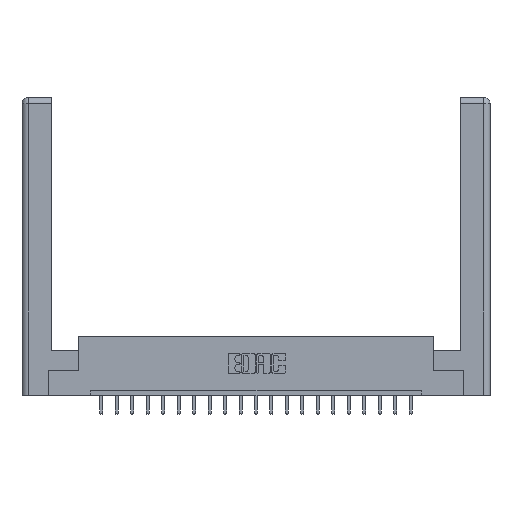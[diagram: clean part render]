
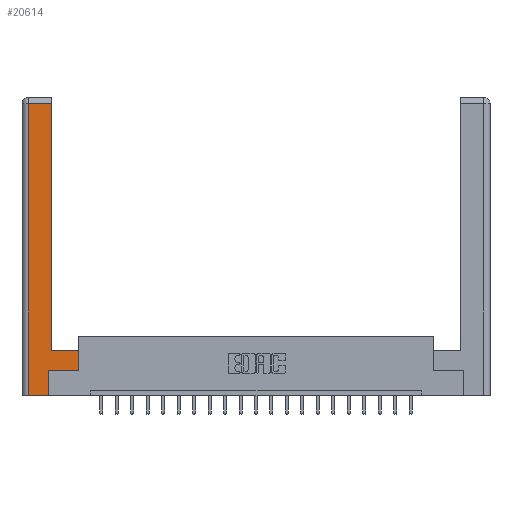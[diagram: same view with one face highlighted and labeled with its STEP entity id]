
A CAD part, top view. The second image highlights one B-rep face of the part: STEP entity #20614.
In plain terms, the highlighted planar face has unit normal (0, 0, 1).
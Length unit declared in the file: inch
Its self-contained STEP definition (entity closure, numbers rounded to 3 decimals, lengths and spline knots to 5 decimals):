
#14 = VERTEX_POINT ( 'NONE', #2744 ) ;
#139 = DIRECTION ( 'NONE',  ( 0., -1., 0. ) ) ;
#161 = LINE ( 'NONE', #10809, #4755 ) ;
#211 = CARTESIAN_POINT ( 'NONE',  ( 0.565, 0.245, 0. ) ) ;
#277 = ORIENTED_EDGE ( 'NONE', *, *, #19937, .T. ) ;
#769 = VERTEX_POINT ( 'NONE', #12745 ) ;
#966 = DIRECTION ( 'NONE',  ( 0., 1., 0. ) ) ;
#1201 = VECTOR ( 'NONE', #10895, 39.37008 ) ;
#1247 = EDGE_CURVE ( 'NONE', #20929, #9600, #13380, .T. ) ;
#1670 = EDGE_LOOP ( 'NONE', ( #7383, #277, #18911, #3865, #18417, #17178, #19690, #11444 ) ) ;
#2225 = VERTEX_POINT ( 'NONE', #3813 ) ;
#2557 = CARTESIAN_POINT ( 'NONE',  ( 0., 0., 0. ) ) ;
#2691 = VECTOR ( 'NONE', #9878, 39.37008 ) ;
#2744 = CARTESIAN_POINT ( 'NONE',  ( 0.0615, 0., 0. ) ) ;
#3380 = CARTESIAN_POINT ( 'NONE',  ( 0.265, 0.245, 0. ) ) ;
#3390 = AXIS2_PLACEMENT_3D ( 'NONE', #2557, #13781, #13850 ) ;
#3813 = CARTESIAN_POINT ( 'NONE',  ( 0.295, 0.45, 0. ) ) ;
#3865 = ORIENTED_EDGE ( 'NONE', *, *, #11251, .T. ) ;
#4700 = VECTOR ( 'NONE', #5051, 39.37008 ) ;
#4755 = VECTOR ( 'NONE', #5991, 39.37008 ) ;
#5001 = CARTESIAN_POINT ( 'NONE',  ( 0.0615, 2.94, 0. ) ) ;
#5007 = LINE ( 'NONE', #20557, #1201 ) ;
#5051 = DIRECTION ( 'NONE',  ( 1., 0., 0. ) ) ;
#5991 = DIRECTION ( 'NONE',  ( 1., 0., 0. ) ) ;
#7077 = DIRECTION ( 'NONE',  ( -1., 0., 0. ) ) ;
#7383 = ORIENTED_EDGE ( 'NONE', *, *, #8585, .T. ) ;
#8111 = EDGE_CURVE ( 'NONE', #16551, #2225, #19938, .T. ) ;
#8377 = CARTESIAN_POINT ( 'NONE',  ( 0.0615, 0., 0. ) ) ;
#8585 = EDGE_CURVE ( 'NONE', #2225, #769, #18625, .T. ) ;
#9307 = LINE ( 'NONE', #8377, #16709 ) ;
#9600 = VERTEX_POINT ( 'NONE', #16632 ) ;
#9878 = DIRECTION ( 'NONE',  ( 0., 1., 0. ) ) ;
#10134 = CARTESIAN_POINT ( 'NONE',  ( 0.265, 0., 0. ) ) ;
#10657 = CARTESIAN_POINT ( 'NONE',  ( 0.565, 0.45, 0. ) ) ;
#10809 = CARTESIAN_POINT ( 'NONE',  ( 0.265, 0., 0. ) ) ;
#10895 = DIRECTION ( 'NONE',  ( -1., 0., 0. ) ) ;
#11251 = EDGE_CURVE ( 'NONE', #14, #20929, #161, .T. ) ;
#11259 = VECTOR ( 'NONE', #7077, 39.37008 ) ;
#11334 = VERTEX_POINT ( 'NONE', #5001 ) ;
#11444 = ORIENTED_EDGE ( 'NONE', *, *, #8111, .T. ) ;
#12060 = LINE ( 'NONE', #211, #4700 ) ;
#12745 = CARTESIAN_POINT ( 'NONE',  ( 0.295, 2.94, 0. ) ) ;
#12782 = VERTEX_POINT ( 'NONE', #14627 ) ;
#13373 = CARTESIAN_POINT ( 'NONE',  ( 0.565, 0.45, 0. ) ) ;
#13380 = LINE ( 'NONE', #3380, #2691 ) ;
#13781 = DIRECTION ( 'NONE',  ( 0., 0., -1. ) ) ;
#13850 = DIRECTION ( 'NONE',  ( -1., 0., 0. ) ) ;
#14519 = LINE ( 'NONE', #10657, #16558 ) ;
#14627 = CARTESIAN_POINT ( 'NONE',  ( 0.565, 0.245, 0. ) ) ;
#14721 = EDGE_CURVE ( 'NONE', #11334, #14, #9307, .T. ) ;
#14874 = FACE_OUTER_BOUND ( 'NONE', #1670, .T. ) ;
#15304 = CARTESIAN_POINT ( 'NONE',  ( 0.295, 0.45, 0. ) ) ;
#15621 = PLANE ( 'NONE',  #3390 ) ;
#16551 = VERTEX_POINT ( 'NONE', #13373 ) ;
#16558 = VECTOR ( 'NONE', #966, 39.37008 ) ;
#16632 = CARTESIAN_POINT ( 'NONE',  ( 0.265, 0.245, 0. ) ) ;
#16709 = VECTOR ( 'NONE', #139, 39.37008 ) ;
#17178 = ORIENTED_EDGE ( 'NONE', *, *, #20819, .T. ) ;
#17513 = EDGE_CURVE ( 'NONE', #12782, #16551, #14519, .T. ) ;
#17585 = VECTOR ( 'NONE', #20465, 39.37008 ) ;
#18417 = ORIENTED_EDGE ( 'NONE', *, *, #1247, .T. ) ;
#18625 = LINE ( 'NONE', #18691, #17585 ) ;
#18691 = CARTESIAN_POINT ( 'NONE',  ( 0.295, 3., 0. ) ) ;
#18911 = ORIENTED_EDGE ( 'NONE', *, *, #14721, .T. ) ;
#19690 = ORIENTED_EDGE ( 'NONE', *, *, #17513, .T. ) ;
#19937 = EDGE_CURVE ( 'NONE', #769, #11334, #5007, .T. ) ;
#19938 = LINE ( 'NONE', #15304, #11259 ) ;
#20465 = DIRECTION ( 'NONE',  ( 0., 1., 0. ) ) ;
#20557 = CARTESIAN_POINT ( 'NONE',  ( 0.0615, 2.94, 0. ) ) ;
#20614 = ADVANCED_FACE ( 'NONE', ( #14874 ), #15621, .F. ) ;
#20819 = EDGE_CURVE ( 'NONE', #9600, #12782, #12060, .T. ) ;
#20929 = VERTEX_POINT ( 'NONE', #10134 ) ;
